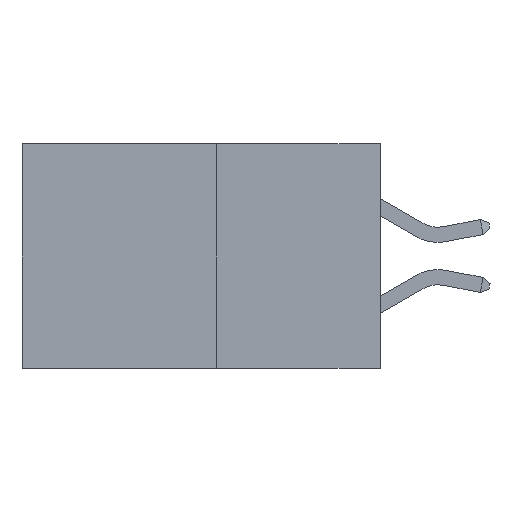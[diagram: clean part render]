
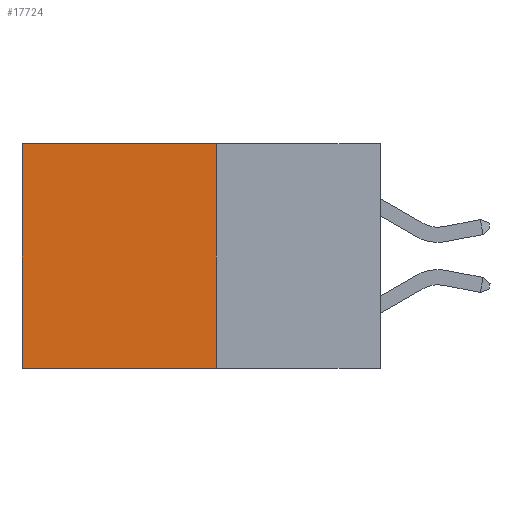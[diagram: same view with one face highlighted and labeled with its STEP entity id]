
A CAD part, left-side view. The second image highlights one B-rep face of the part: STEP entity #17724.
In plain terms, the highlighted planar face has unit normal (-1, 0, 0).
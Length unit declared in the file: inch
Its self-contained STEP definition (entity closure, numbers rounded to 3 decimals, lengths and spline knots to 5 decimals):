
#1307 = VERTEX_POINT ( 'NONE', #19884 ) ;
#2105 = CARTESIAN_POINT ( 'NONE',  ( 0.277, 0.27, -0.37 ) ) ;
#3040 = PLANE ( 'NONE',  #15957 ) ;
#3798 = LINE ( 'NONE', #6697, #8199 ) ;
#3855 = EDGE_CURVE ( 'NONE', #15847, #1307, #3798, .T. ) ;
#4554 = LINE ( 'NONE', #2105, #12710 ) ;
#4949 = DIRECTION ( 'NONE',  ( 0., 0., -1. ) ) ;
#6697 = CARTESIAN_POINT ( 'NONE',  ( 0.277, 0.59, -0.37 ) ) ;
#6778 = DIRECTION ( 'NONE',  ( 0., 0., -1. ) ) ;
#7090 = EDGE_CURVE ( 'NONE', #12643, #1307, #22272, .T. ) ;
#7435 = VECTOR ( 'NONE', #16344, 39.37008 ) ;
#8199 = VECTOR ( 'NONE', #6778, 39.37008 ) ;
#9172 = VECTOR ( 'NONE', #15595, 39.37008 ) ;
#9389 = CARTESIAN_POINT ( 'NONE',  ( 0.277, 0.27, -0.37 ) ) ;
#9467 = DIRECTION ( 'NONE',  ( 0., 0., -1. ) ) ;
#9860 = ORIENTED_EDGE ( 'NONE', *, *, #12702, .F. ) ;
#10732 = ORIENTED_EDGE ( 'NONE', *, *, #3855, .T. ) ;
#11421 = VERTEX_POINT ( 'NONE', #11644 ) ;
#11644 = CARTESIAN_POINT ( 'NONE',  ( 0.277, 0.27, 0. ) ) ;
#12643 = VERTEX_POINT ( 'NONE', #9389 ) ;
#12702 = EDGE_CURVE ( 'NONE', #11421, #12643, #4554, .T. ) ;
#12710 = VECTOR ( 'NONE', #9467, 39.37008 ) ;
#13707 = CARTESIAN_POINT ( 'NONE',  ( 0.277, 0.27, 0. ) ) ;
#14047 = EDGE_CURVE ( 'NONE', #11421, #15847, #14103, .T. ) ;
#14103 = LINE ( 'NONE', #13707, #9172 ) ;
#15595 = DIRECTION ( 'NONE',  ( 0., 1., 0. ) ) ;
#15847 = VERTEX_POINT ( 'NONE', #22013 ) ;
#15957 = AXIS2_PLACEMENT_3D ( 'NONE', #19832, #16140, #4949 ) ;
#16140 = DIRECTION ( 'NONE',  ( 1., 0., 0. ) ) ;
#16263 = CARTESIAN_POINT ( 'NONE',  ( 0.277, 0.27, -0.37 ) ) ;
#16344 = DIRECTION ( 'NONE',  ( 0., 1., 0. ) ) ;
#17000 = ORIENTED_EDGE ( 'NONE', *, *, #14047, .T. ) ;
#17724 = ADVANCED_FACE ( 'NONE', ( #22467 ), #3040, .F. ) ;
#17876 = ORIENTED_EDGE ( 'NONE', *, *, #7090, .F. ) ;
#19832 = CARTESIAN_POINT ( 'NONE',  ( 0.277, 0.27, -0.37 ) ) ;
#19884 = CARTESIAN_POINT ( 'NONE',  ( 0.277, 0.59, -0.37 ) ) ;
#21562 = EDGE_LOOP ( 'NONE', ( #10732, #17876, #9860, #17000 ) ) ;
#22013 = CARTESIAN_POINT ( 'NONE',  ( 0.277, 0.59, 0. ) ) ;
#22272 = LINE ( 'NONE', #16263, #7435 ) ;
#22467 = FACE_OUTER_BOUND ( 'NONE', #21562, .T. ) ;
